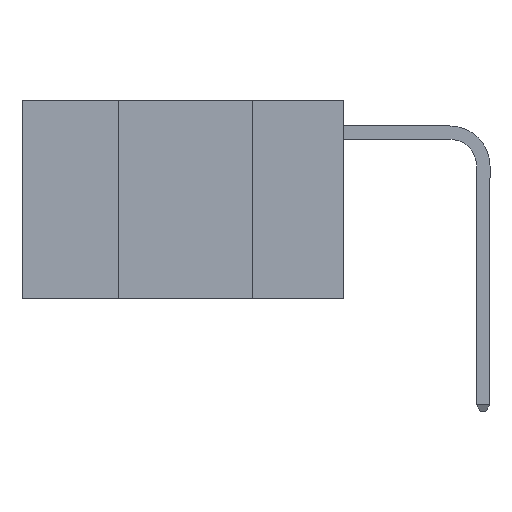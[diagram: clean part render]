
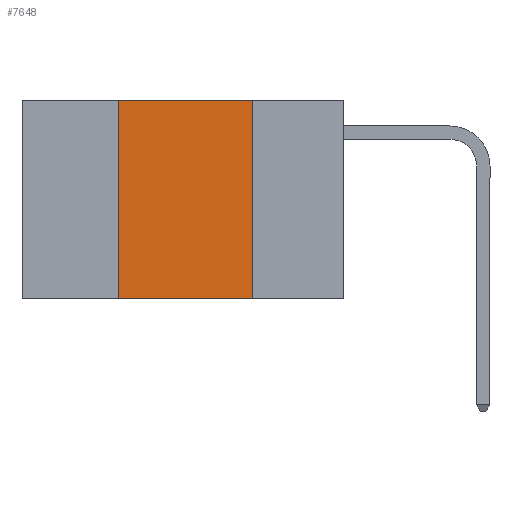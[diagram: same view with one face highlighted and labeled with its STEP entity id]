
A CAD part, left-side view. The second image highlights one B-rep face of the part: STEP entity #7648.
In plain terms, the highlighted planar face has unit normal (-1, 0, 0).
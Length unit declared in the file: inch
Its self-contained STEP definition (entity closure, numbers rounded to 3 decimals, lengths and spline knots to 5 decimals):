
#491 = LINE ( 'NONE', #4671, #6997 ) ;
#499 = CARTESIAN_POINT ( 'NONE',  ( 0., 0.17, 0. ) ) ;
#954 = EDGE_CURVE ( 'NONE', #13265, #8204, #11064, .T. ) ;
#1446 = DIRECTION ( 'NONE',  ( 0., 0., -1. ) ) ;
#1845 = VERTEX_POINT ( 'NONE', #6574 ) ;
#2454 = DIRECTION ( 'NONE',  ( 0., 0., 1. ) ) ;
#2527 = VERTEX_POINT ( 'NONE', #16436 ) ;
#2536 = ORIENTED_EDGE ( 'NONE', *, *, #12013, .F. ) ;
#2564 = EDGE_CURVE ( 'NONE', #13265, #1845, #491, .T. ) ;
#3206 = LINE ( 'NONE', #499, #12677 ) ;
#4671 = CARTESIAN_POINT ( 'NONE',  ( 0., 0.42, 0. ) ) ;
#5473 = FACE_OUTER_BOUND ( 'NONE', #10889, .T. ) ;
#6574 = CARTESIAN_POINT ( 'NONE',  ( 0., 0.42, 0. ) ) ;
#6608 = PLANE ( 'NONE',  #12908 ) ;
#6782 = ORIENTED_EDGE ( 'NONE', *, *, #2564, .F. ) ;
#6997 = VECTOR ( 'NONE', #2454, 39.37008 ) ;
#7648 = ADVANCED_FACE ( 'NONE', ( #5473 ), #6608, .F. ) ;
#8204 = VERTEX_POINT ( 'NONE', #10347 ) ;
#8653 = CARTESIAN_POINT ( 'NONE',  ( 0., 0.6, 0. ) ) ;
#9194 = DIRECTION ( 'NONE',  ( 1., 0., 0. ) ) ;
#9948 = DIRECTION ( 'NONE',  ( 0., -1., 0. ) ) ;
#10139 = CARTESIAN_POINT ( 'NONE',  ( 0., 0.42, -0.37 ) ) ;
#10347 = CARTESIAN_POINT ( 'NONE',  ( 0., 0.17, -0.37 ) ) ;
#10889 = EDGE_LOOP ( 'NONE', ( #12430, #2536, #6782, #13605 ) ) ;
#11064 = LINE ( 'NONE', #16030, #14825 ) ;
#11558 = VECTOR ( 'NONE', #9948, 39.37008 ) ;
#11721 = LINE ( 'NONE', #8653, #11558 ) ;
#12013 = EDGE_CURVE ( 'NONE', #1845, #2527, #11721, .T. ) ;
#12430 = ORIENTED_EDGE ( 'NONE', *, *, #13642, .F. ) ;
#12677 = VECTOR ( 'NONE', #13440, 39.37008 ) ;
#12908 = AXIS2_PLACEMENT_3D ( 'NONE', #13023, #9194, #1446 ) ;
#12931 = DIRECTION ( 'NONE',  ( 0., -1., 0. ) ) ;
#13023 = CARTESIAN_POINT ( 'NONE',  ( 0., 0.6, 0. ) ) ;
#13265 = VERTEX_POINT ( 'NONE', #10139 ) ;
#13440 = DIRECTION ( 'NONE',  ( 0., 0., -1. ) ) ;
#13605 = ORIENTED_EDGE ( 'NONE', *, *, #954, .T. ) ;
#13642 = EDGE_CURVE ( 'NONE', #2527, #8204, #3206, .T. ) ;
#14825 = VECTOR ( 'NONE', #12931, 39.37008 ) ;
#16030 = CARTESIAN_POINT ( 'NONE',  ( 0., 0.6, -0.37 ) ) ;
#16436 = CARTESIAN_POINT ( 'NONE',  ( 0., 0.17, 0. ) ) ;
